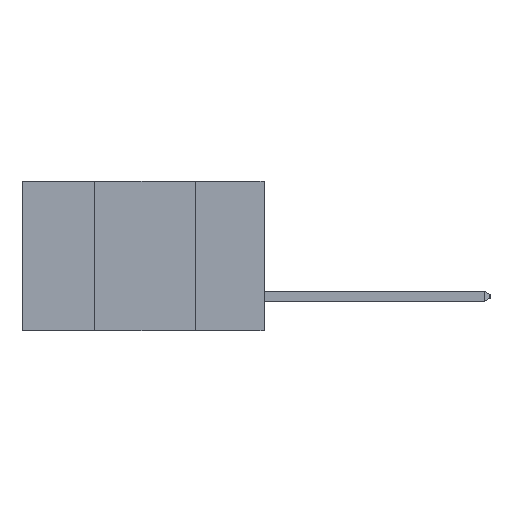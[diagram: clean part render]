
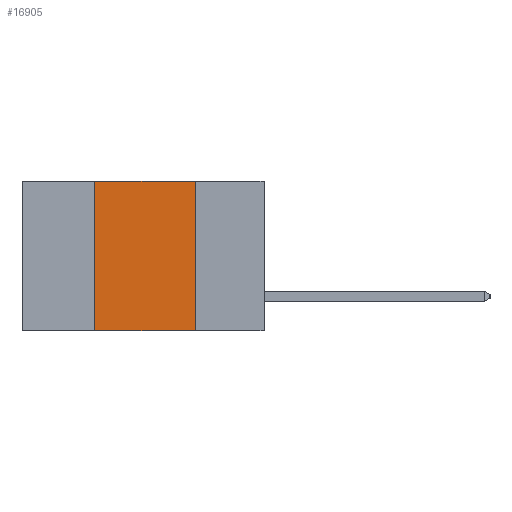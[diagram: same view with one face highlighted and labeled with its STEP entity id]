
A CAD part, left-side view. The second image highlights one B-rep face of the part: STEP entity #16905.
In plain terms, the highlighted planar face has unit normal (-1, 0, 0).
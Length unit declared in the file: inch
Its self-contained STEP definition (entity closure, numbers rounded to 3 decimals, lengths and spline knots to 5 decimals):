
#517 = ORIENTED_EDGE ( 'NONE', *, *, #3134, .F. ) ;
#1243 = CARTESIAN_POINT ( 'NONE',  ( 0., 0.42, -0.37 ) ) ;
#1382 = CARTESIAN_POINT ( 'NONE',  ( 0., 0.6, 0. ) ) ;
#1738 = ORIENTED_EDGE ( 'NONE', *, *, #21081, .F. ) ;
#2288 = VECTOR ( 'NONE', #8818, 39.37008 ) ;
#3134 = EDGE_CURVE ( 'NONE', #11960, #16765, #21525, .T. ) ;
#3283 = EDGE_LOOP ( 'NONE', ( #6764, #1738, #517, #14445 ) ) ;
#3290 = VECTOR ( 'NONE', #11948, 39.37008 ) ;
#3325 = DIRECTION ( 'NONE',  ( 0., -1., 0. ) ) ;
#4864 = LINE ( 'NONE', #1382, #23058 ) ;
#6764 = ORIENTED_EDGE ( 'NONE', *, *, #14356, .F. ) ;
#7282 = LINE ( 'NONE', #12554, #2288 ) ;
#8068 = CARTESIAN_POINT ( 'NONE',  ( 0., 0.42, 0. ) ) ;
#8818 = DIRECTION ( 'NONE',  ( 0., -1., 0. ) ) ;
#10289 = CARTESIAN_POINT ( 'NONE',  ( 0., 0.6, 0. ) ) ;
#11614 = CARTESIAN_POINT ( 'NONE',  ( 0., 0.17, -0.37 ) ) ;
#11629 = VERTEX_POINT ( 'NONE', #11614 ) ;
#11948 = DIRECTION ( 'NONE',  ( 0., 0., 1. ) ) ;
#11960 = VERTEX_POINT ( 'NONE', #1243 ) ;
#12227 = DIRECTION ( 'NONE',  ( 0., 0., -1. ) ) ;
#12554 = CARTESIAN_POINT ( 'NONE',  ( 0., 0.6, -0.37 ) ) ;
#14319 = AXIS2_PLACEMENT_3D ( 'NONE', #10289, #23412, #12227 ) ;
#14356 = EDGE_CURVE ( 'NONE', #22638, #11629, #24208, .T. ) ;
#14445 = ORIENTED_EDGE ( 'NONE', *, *, #18567, .T. ) ;
#15750 = CARTESIAN_POINT ( 'NONE',  ( 0., 0.42, -0.37 ) ) ;
#16765 = VERTEX_POINT ( 'NONE', #8068 ) ;
#16905 = ADVANCED_FACE ( 'NONE', ( #22388 ), #23334, .F. ) ;
#17893 = CARTESIAN_POINT ( 'NONE',  ( 0., 0.17, -0.37 ) ) ;
#18567 = EDGE_CURVE ( 'NONE', #11960, #11629, #7282, .T. ) ;
#19326 = VECTOR ( 'NONE', #20788, 39.37008 ) ;
#20788 = DIRECTION ( 'NONE',  ( 0., 0., -1. ) ) ;
#20948 = CARTESIAN_POINT ( 'NONE',  ( 0., 0.17, 0. ) ) ;
#21081 = EDGE_CURVE ( 'NONE', #16765, #22638, #4864, .T. ) ;
#21525 = LINE ( 'NONE', #15750, #3290 ) ;
#22388 = FACE_OUTER_BOUND ( 'NONE', #3283, .T. ) ;
#22638 = VERTEX_POINT ( 'NONE', #20948 ) ;
#23058 = VECTOR ( 'NONE', #3325, 39.37008 ) ;
#23334 = PLANE ( 'NONE',  #14319 ) ;
#23412 = DIRECTION ( 'NONE',  ( 1., 0., 0. ) ) ;
#24208 = LINE ( 'NONE', #17893, #19326 ) ;
